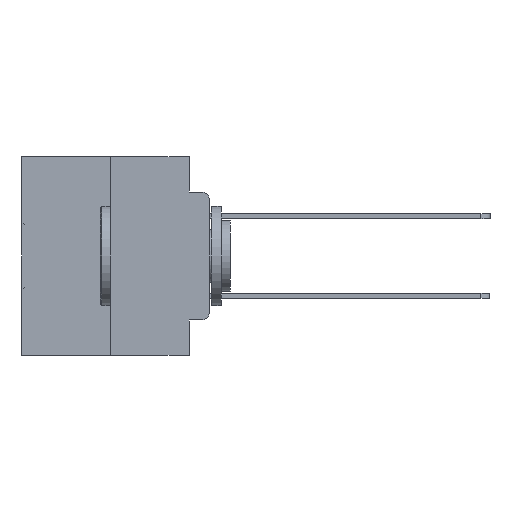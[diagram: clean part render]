
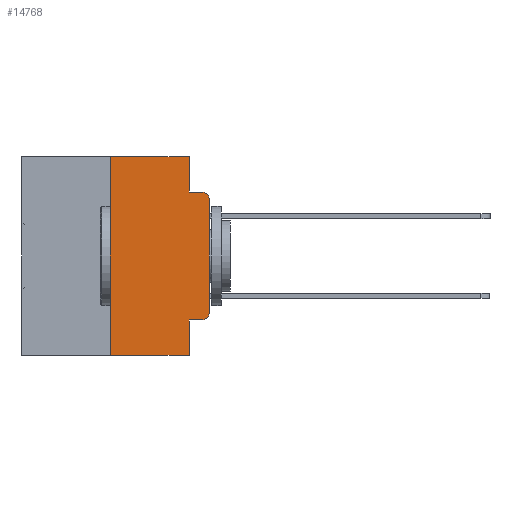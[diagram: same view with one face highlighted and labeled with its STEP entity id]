
A CAD part, left-side view. The second image highlights one B-rep face of the part: STEP entity #14768.
In plain terms, the highlighted planar face has unit normal (-1, 0, 0).
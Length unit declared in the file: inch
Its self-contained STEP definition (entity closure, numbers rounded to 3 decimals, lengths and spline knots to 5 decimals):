
#278 = VERTEX_POINT ( 'NONE', #29429 ) ;
#285 = VERTEX_POINT ( 'NONE', #14226 ) ;
#422 = CARTESIAN_POINT ( 'NONE',  ( 0., 0.02, -0.4115 ) ) ;
#960 = VERTEX_POINT ( 'NONE', #12727 ) ;
#1630 = DIRECTION ( 'NONE',  ( 0., -1., 0. ) ) ;
#1920 = VERTEX_POINT ( 'NONE', #23415 ) ;
#2873 = VECTOR ( 'NONE', #4165, 39.37008 ) ;
#3127 = LINE ( 'NONE', #24371, #15046 ) ;
#3255 = EDGE_CURVE ( 'NONE', #17827, #11962, #28674, .T. ) ;
#3602 = EDGE_LOOP ( 'NONE', ( #23160, #10460, #4514, #18042, #32012, #12869, #15260, #9247, #10873, #30875 ) ) ;
#4075 = FACE_OUTER_BOUND ( 'NONE', #3602, .T. ) ;
#4165 = DIRECTION ( 'NONE',  ( 0., 0., 1. ) ) ;
#4514 = ORIENTED_EDGE ( 'NONE', *, *, #4972, .F. ) ;
#4972 = EDGE_CURVE ( 'NONE', #11962, #30573, #12907, .T. ) ;
#5310 = CARTESIAN_POINT ( 'NONE',  ( 0., 0.02, -0.1085 ) ) ;
#6630 = CARTESIAN_POINT ( 'NONE',  ( 0., 0.02, -0.0885 ) ) ;
#7851 = DIRECTION ( 'NONE',  ( 0., 0., -1. ) ) ;
#8106 = DIRECTION ( 'NONE',  ( 1., 0., 0. ) ) ;
#8172 = AXIS2_PLACEMENT_3D ( 'NONE', #23325, #8106, #25813 ) ;
#8333 = EDGE_CURVE ( 'NONE', #285, #30573, #19041, .T. ) ;
#8578 = CARTESIAN_POINT ( 'NONE',  ( 0., 0.02, -0.3915 ) ) ;
#8665 = DIRECTION ( 'NONE',  ( 0., 0., -1. ) ) ;
#9247 = ORIENTED_EDGE ( 'NONE', *, *, #25946, .F. ) ;
#9392 = VECTOR ( 'NONE', #14068, 39.37008 ) ;
#9996 = CARTESIAN_POINT ( 'NONE',  ( 0., 0.051, -0.0885 ) ) ;
#10460 = ORIENTED_EDGE ( 'NONE', *, *, #8333, .T. ) ;
#10873 = ORIENTED_EDGE ( 'NONE', *, *, #24279, .T. ) ;
#11159 = DIRECTION ( 'NONE',  ( 0., 0., -1. ) ) ;
#11397 = CARTESIAN_POINT ( 'NONE',  ( 0., 0.051, -0.4115 ) ) ;
#11536 = CARTESIAN_POINT ( 'NONE',  ( 0., 0.473, 0. ) ) ;
#11562 = CIRCLE ( 'NONE', #18327, 0.02 ) ;
#11962 = VERTEX_POINT ( 'NONE', #9996 ) ;
#12208 = VERTEX_POINT ( 'NONE', #30941 ) ;
#12267 = VERTEX_POINT ( 'NONE', #21327 ) ;
#12727 = CARTESIAN_POINT ( 'NONE',  ( 0., 0.051, -0.4115 ) ) ;
#12869 = ORIENTED_EDGE ( 'NONE', *, *, #27591, .F. ) ;
#12907 = LINE ( 'NONE', #18485, #32048 ) ;
#13340 = LINE ( 'NONE', #17610, #25974 ) ;
#13923 = DIRECTION ( 'NONE',  ( 0., -1., 0. ) ) ;
#14068 = DIRECTION ( 'NONE',  ( 0., -1., 0. ) ) ;
#14226 = CARTESIAN_POINT ( 'NONE',  ( 0., 0., -0.1085 ) ) ;
#14756 = DIRECTION ( 'NONE',  ( 0., 0., 1. ) ) ;
#14768 = ADVANCED_FACE ( 'NONE', ( #4075 ), #18150, .F. ) ;
#15046 = VECTOR ( 'NONE', #1630, 39.37008 ) ;
#15191 = EDGE_CURVE ( 'NONE', #12208, #285, #26877, .T. ) ;
#15260 = ORIENTED_EDGE ( 'NONE', *, *, #15617, .T. ) ;
#15358 = VECTOR ( 'NONE', #8665, 39.37008 ) ;
#15445 = VECTOR ( 'NONE', #13923, 39.37008 ) ;
#15601 = LINE ( 'NONE', #19402, #2873 ) ;
#15617 = EDGE_CURVE ( 'NONE', #12267, #1920, #3127, .T. ) ;
#16236 = LINE ( 'NONE', #11397, #15445 ) ;
#17610 = CARTESIAN_POINT ( 'NONE',  ( 0., 0.051, 0. ) ) ;
#17827 = VERTEX_POINT ( 'NONE', #20814 ) ;
#18042 = ORIENTED_EDGE ( 'NONE', *, *, #3255, .F. ) ;
#18150 = PLANE ( 'NONE',  #8172 ) ;
#18327 = AXIS2_PLACEMENT_3D ( 'NONE', #8578, #26280, #11159 ) ;
#18485 = CARTESIAN_POINT ( 'NONE',  ( 0., 0.051, -0.0885 ) ) ;
#19041 = CIRCLE ( 'NONE', #23785, 0.02 ) ;
#19402 = CARTESIAN_POINT ( 'NONE',  ( 0., 0.25, 0. ) ) ;
#20177 = DIRECTION ( 'NONE',  ( 0., 0., -1. ) ) ;
#20257 = VECTOR ( 'NONE', #14756, 39.37008 ) ;
#20814 = CARTESIAN_POINT ( 'NONE',  ( 0., 0.051, 0. ) ) ;
#20928 = EDGE_CURVE ( 'NONE', #27947, #12208, #11562, .T. ) ;
#21327 = CARTESIAN_POINT ( 'NONE',  ( 0., 0.25, -0.5 ) ) ;
#23068 = DIRECTION ( 'NONE',  ( -1., 0., 0. ) ) ;
#23160 = ORIENTED_EDGE ( 'NONE', *, *, #15191, .T. ) ;
#23325 = CARTESIAN_POINT ( 'NONE',  ( 0., 0.473, 0. ) ) ;
#23415 = CARTESIAN_POINT ( 'NONE',  ( 0., 0.051, -0.5 ) ) ;
#23785 = AXIS2_PLACEMENT_3D ( 'NONE', #5310, #23068, #7851 ) ;
#24279 = EDGE_CURVE ( 'NONE', #960, #27947, #16236, .T. ) ;
#24371 = CARTESIAN_POINT ( 'NONE',  ( 0., 0.473, -0.5 ) ) ;
#25813 = DIRECTION ( 'NONE',  ( 0., 0., -1. ) ) ;
#25926 = DIRECTION ( 'NONE',  ( 0., -1., 0. ) ) ;
#25946 = EDGE_CURVE ( 'NONE', #960, #1920, #13340, .T. ) ;
#25974 = VECTOR ( 'NONE', #20177, 39.37008 ) ;
#26280 = DIRECTION ( 'NONE',  ( -1., 0., 0. ) ) ;
#26877 = LINE ( 'NONE', #27295, #20257 ) ;
#27295 = CARTESIAN_POINT ( 'NONE',  ( 0., 0., 0. ) ) ;
#27591 = EDGE_CURVE ( 'NONE', #12267, #278, #15601, .T. ) ;
#27947 = VERTEX_POINT ( 'NONE', #422 ) ;
#28674 = LINE ( 'NONE', #31295, #15358 ) ;
#29429 = CARTESIAN_POINT ( 'NONE',  ( 0., 0.25, 0. ) ) ;
#29486 = LINE ( 'NONE', #11536, #9392 ) ;
#30485 = EDGE_CURVE ( 'NONE', #278, #17827, #29486, .T. ) ;
#30573 = VERTEX_POINT ( 'NONE', #6630 ) ;
#30875 = ORIENTED_EDGE ( 'NONE', *, *, #20928, .T. ) ;
#30941 = CARTESIAN_POINT ( 'NONE',  ( 0., 0., -0.3915 ) ) ;
#31295 = CARTESIAN_POINT ( 'NONE',  ( 0., 0.051, 0. ) ) ;
#32012 = ORIENTED_EDGE ( 'NONE', *, *, #30485, .F. ) ;
#32048 = VECTOR ( 'NONE', #25926, 39.37008 ) ;
